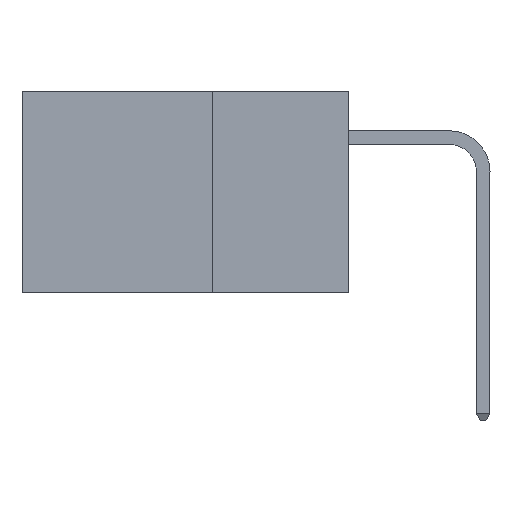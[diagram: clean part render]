
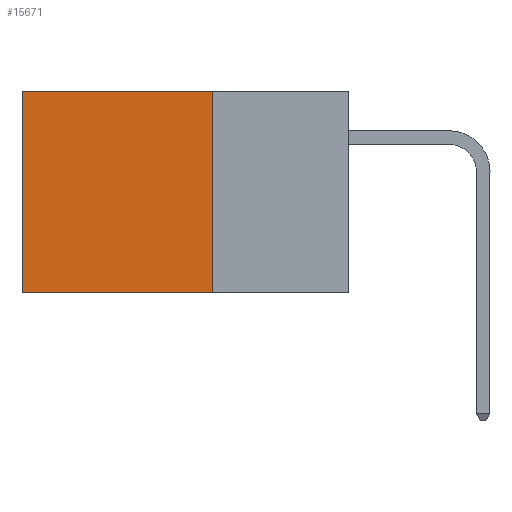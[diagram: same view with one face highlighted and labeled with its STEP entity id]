
A CAD part, left-side view. The second image highlights one B-rep face of the part: STEP entity #15671.
In plain terms, the highlighted planar face has unit normal (-1, 0, 0).
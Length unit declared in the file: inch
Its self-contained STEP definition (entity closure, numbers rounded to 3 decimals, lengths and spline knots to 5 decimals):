
#752 = CARTESIAN_POINT ( 'NONE',  ( 0.2875, 0.25, 0. ) ) ;
#783 = VERTEX_POINT ( 'NONE', #5307 ) ;
#1867 = CARTESIAN_POINT ( 'NONE',  ( 0.2875, 0.25, 0. ) ) ;
#2248 = CARTESIAN_POINT ( 'NONE',  ( 0.2875, 0.25, 0. ) ) ;
#2275 = ORIENTED_EDGE ( 'NONE', *, *, #11738, .F. ) ;
#2887 = LINE ( 'NONE', #4280, #9192 ) ;
#3275 = EDGE_CURVE ( 'NONE', #14420, #783, #2887, .T. ) ;
#3616 = DIRECTION ( 'NONE',  ( 0., 0., -1. ) ) ;
#4201 = CARTESIAN_POINT ( 'NONE',  ( 0.2875, 0.6, 0. ) ) ;
#4280 = CARTESIAN_POINT ( 'NONE',  ( 0.2875, 0.25, -0.37 ) ) ;
#4324 = ORIENTED_EDGE ( 'NONE', *, *, #14343, .T. ) ;
#5189 = VECTOR ( 'NONE', #16686, 39.37008 ) ;
#5307 = CARTESIAN_POINT ( 'NONE',  ( 0.2875, 0.6, -0.37 ) ) ;
#5592 = LINE ( 'NONE', #1867, #5189 ) ;
#5892 = EDGE_LOOP ( 'NONE', ( #4324, #6744, #2275, #6257 ) ) ;
#6185 = LINE ( 'NONE', #2248, #9773 ) ;
#6257 = ORIENTED_EDGE ( 'NONE', *, *, #8403, .T. ) ;
#6570 = DIRECTION ( 'NONE',  ( 1., 0., 0. ) ) ;
#6744 = ORIENTED_EDGE ( 'NONE', *, *, #3275, .F. ) ;
#6983 = CARTESIAN_POINT ( 'NONE',  ( 0.2875, 0.25, -0.37 ) ) ;
#7825 = VERTEX_POINT ( 'NONE', #12761 ) ;
#8165 = DIRECTION ( 'NONE',  ( 0., 0., -1. ) ) ;
#8303 = DIRECTION ( 'NONE',  ( 0., 1., 0. ) ) ;
#8403 = EDGE_CURVE ( 'NONE', #12316, #7825, #5592, .T. ) ;
#9192 = VECTOR ( 'NONE', #8303, 39.37008 ) ;
#9236 = CARTESIAN_POINT ( 'NONE',  ( 0.2875, 0.25, 0. ) ) ;
#9299 = AXIS2_PLACEMENT_3D ( 'NONE', #9236, #6570, #15999 ) ;
#9773 = VECTOR ( 'NONE', #3616, 39.37008 ) ;
#9810 = LINE ( 'NONE', #4201, #16970 ) ;
#11738 = EDGE_CURVE ( 'NONE', #12316, #14420, #6185, .T. ) ;
#11958 = PLANE ( 'NONE',  #9299 ) ;
#12316 = VERTEX_POINT ( 'NONE', #752 ) ;
#12761 = CARTESIAN_POINT ( 'NONE',  ( 0.2875, 0.6, 0. ) ) ;
#14343 = EDGE_CURVE ( 'NONE', #7825, #783, #9810, .T. ) ;
#14420 = VERTEX_POINT ( 'NONE', #6983 ) ;
#15671 = ADVANCED_FACE ( 'NONE', ( #16490 ), #11958, .F. ) ;
#15999 = DIRECTION ( 'NONE',  ( 0., 0., -1. ) ) ;
#16490 = FACE_OUTER_BOUND ( 'NONE', #5892, .T. ) ;
#16686 = DIRECTION ( 'NONE',  ( 0., 1., 0. ) ) ;
#16970 = VECTOR ( 'NONE', #8165, 39.37008 ) ;
